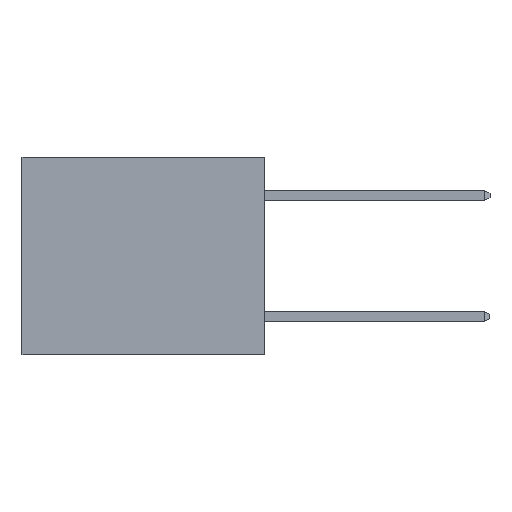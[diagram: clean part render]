
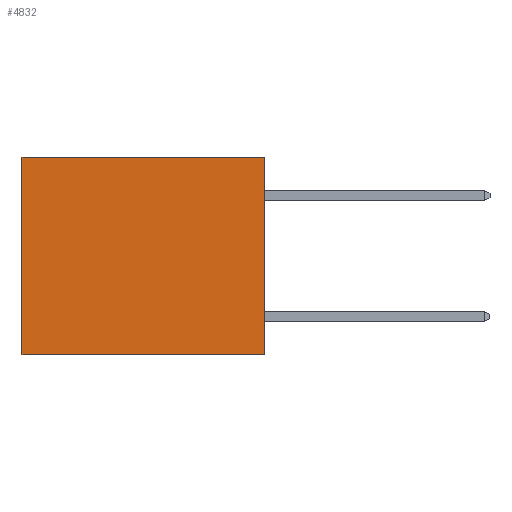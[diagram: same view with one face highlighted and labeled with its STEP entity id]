
A CAD part, left-side view. The second image highlights one B-rep face of the part: STEP entity #4832.
In plain terms, the highlighted planar face has unit normal (-1, 0, 0).
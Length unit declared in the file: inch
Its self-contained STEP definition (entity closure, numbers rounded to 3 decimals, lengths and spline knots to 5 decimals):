
#644 = CARTESIAN_POINT ( 'NONE',  ( 0.3165, 0., -0.49 ) ) ;
#1322 = VERTEX_POINT ( 'NONE', #6996 ) ;
#1728 = CARTESIAN_POINT ( 'NONE',  ( 0.3165, 0.6, -0.49 ) ) ;
#1739 = EDGE_CURVE ( 'NONE', #1322, #8034, #6548, .T. ) ;
#1988 = CARTESIAN_POINT ( 'NONE',  ( 0.3165, 0., -0.49 ) ) ;
#2151 = CARTESIAN_POINT ( 'NONE',  ( 0.3165, 0., 0. ) ) ;
#3202 = CARTESIAN_POINT ( 'NONE',  ( 0.3165, 0., 0. ) ) ;
#3669 = DIRECTION ( 'NONE',  ( 0., 0., -1. ) ) ;
#4832 = ADVANCED_FACE ( 'NONE', ( #13392 ), #10249, .F. ) ;
#5606 = CARTESIAN_POINT ( 'NONE',  ( 0.3165, 0., -0.49 ) ) ;
#6068 = CARTESIAN_POINT ( 'NONE',  ( 0.3165, 0., -0.49 ) ) ;
#6176 = DIRECTION ( 'NONE',  ( 0., 1., 0. ) ) ;
#6548 = LINE ( 'NONE', #13284, #13102 ) ;
#6996 = CARTESIAN_POINT ( 'NONE',  ( 0.3165, 0.6, 0. ) ) ;
#7824 = AXIS2_PLACEMENT_3D ( 'NONE', #1988, #11717, #13840 ) ;
#7903 = EDGE_CURVE ( 'NONE', #12096, #8034, #12204, .T. ) ;
#8034 = VERTEX_POINT ( 'NONE', #1728 ) ;
#8089 = ORIENTED_EDGE ( 'NONE', *, *, #13687, .T. ) ;
#8349 = DIRECTION ( 'NONE',  ( 0., 1., 0. ) ) ;
#9146 = VECTOR ( 'NONE', #10362, 39.37008 ) ;
#9252 = EDGE_CURVE ( 'NONE', #13306, #12096, #12000, .T. ) ;
#9999 = EDGE_LOOP ( 'NONE', ( #12393, #13070, #10998, #8089 ) ) ;
#10249 = PLANE ( 'NONE',  #7824 ) ;
#10362 = DIRECTION ( 'NONE',  ( 0., 0., -1. ) ) ;
#10998 = ORIENTED_EDGE ( 'NONE', *, *, #9252, .F. ) ;
#11717 = DIRECTION ( 'NONE',  ( 1., 0., 0. ) ) ;
#12000 = LINE ( 'NONE', #644, #9146 ) ;
#12096 = VERTEX_POINT ( 'NONE', #5606 ) ;
#12204 = LINE ( 'NONE', #6068, #13055 ) ;
#12393 = ORIENTED_EDGE ( 'NONE', *, *, #1739, .T. ) ;
#13031 = VECTOR ( 'NONE', #8349, 39.37008 ) ;
#13055 = VECTOR ( 'NONE', #6176, 39.37008 ) ;
#13070 = ORIENTED_EDGE ( 'NONE', *, *, #7903, .F. ) ;
#13102 = VECTOR ( 'NONE', #3669, 39.37008 ) ;
#13284 = CARTESIAN_POINT ( 'NONE',  ( 0.3165, 0.6, -0.49 ) ) ;
#13306 = VERTEX_POINT ( 'NONE', #2151 ) ;
#13392 = FACE_OUTER_BOUND ( 'NONE', #9999, .T. ) ;
#13687 = EDGE_CURVE ( 'NONE', #13306, #1322, #13874, .T. ) ;
#13840 = DIRECTION ( 'NONE',  ( 0., 0., -1. ) ) ;
#13874 = LINE ( 'NONE', #3202, #13031 ) ;
